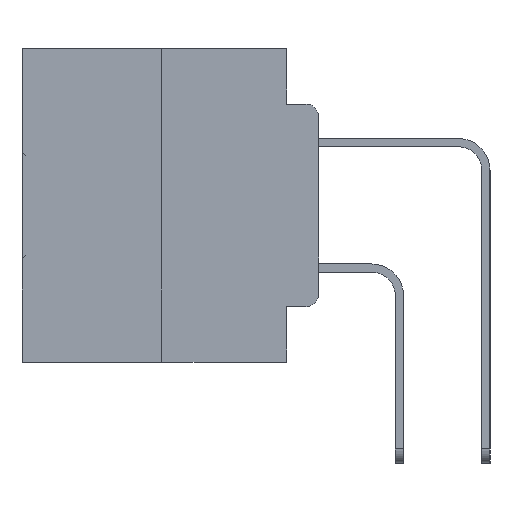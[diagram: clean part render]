
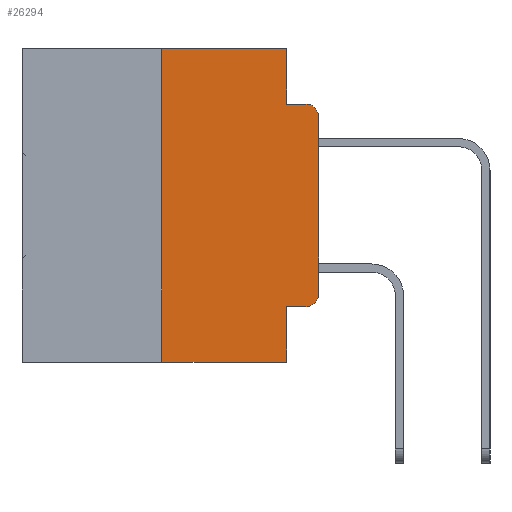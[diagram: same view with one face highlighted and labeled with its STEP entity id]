
A CAD part, left-side view. The second image highlights one B-rep face of the part: STEP entity #26294.
In plain terms, the highlighted planar face has unit normal (-1, 0, 0).
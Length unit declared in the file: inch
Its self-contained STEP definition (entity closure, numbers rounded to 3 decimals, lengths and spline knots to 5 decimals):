
#323 = CARTESIAN_POINT ( 'NONE',  ( 0., 0.02, -0.4115 ) ) ;
#711 = DIRECTION ( 'NONE',  ( 0., 0., -1. ) ) ;
#978 = VERTEX_POINT ( 'NONE', #22649 ) ;
#1404 = EDGE_CURVE ( 'NONE', #21995, #10503, #4610, .T. ) ;
#1432 = EDGE_CURVE ( 'NONE', #27067, #14574, #30393, .T. ) ;
#1796 = CARTESIAN_POINT ( 'NONE',  ( 0., 0.02, -0.3915 ) ) ;
#3207 = ORIENTED_EDGE ( 'NONE', *, *, #8226, .T. ) ;
#3226 = PLANE ( 'NONE',  #10144 ) ;
#4216 = DIRECTION ( 'NONE',  ( 0., -1., 0. ) ) ;
#4441 = DIRECTION ( 'NONE',  ( 0., 0., -1. ) ) ;
#4610 = LINE ( 'NONE', #26064, #17770 ) ;
#4712 = DIRECTION ( 'NONE',  ( 0., 0., -1. ) ) ;
#5640 = CARTESIAN_POINT ( 'NONE',  ( 0., 0., 0. ) ) ;
#6127 = ORIENTED_EDGE ( 'NONE', *, *, #20024, .F. ) ;
#6756 = CARTESIAN_POINT ( 'NONE',  ( 0., 0.473, 0. ) ) ;
#6758 = VECTOR ( 'NONE', #10884, 39.37008 ) ;
#6919 = VECTOR ( 'NONE', #30188, 39.37008 ) ;
#8086 = CARTESIAN_POINT ( 'NONE',  ( 0., 0.25, -0.5 ) ) ;
#8226 = EDGE_CURVE ( 'NONE', #978, #9316, #20683, .T. ) ;
#9015 = CARTESIAN_POINT ( 'NONE',  ( 0., 0.051, -0.4115 ) ) ;
#9114 = CIRCLE ( 'NONE', #15285, 0.02 ) ;
#9316 = VERTEX_POINT ( 'NONE', #19283 ) ;
#9957 = CARTESIAN_POINT ( 'NONE',  ( 0., 0.051, 0. ) ) ;
#10144 = AXIS2_PLACEMENT_3D ( 'NONE', #31971, #16475, #711 ) ;
#10295 = EDGE_CURVE ( 'NONE', #32346, #23845, #12346, .T. ) ;
#10503 = VERTEX_POINT ( 'NONE', #24082 ) ;
#10884 = DIRECTION ( 'NONE',  ( 0., 0., 1. ) ) ;
#10976 = EDGE_CURVE ( 'NONE', #27067, #10503, #20501, .T. ) ;
#11016 = CIRCLE ( 'NONE', #32434, 0.02 ) ;
#11503 = EDGE_CURVE ( 'NONE', #14574, #978, #11016, .T. ) ;
#11530 = VECTOR ( 'NONE', #15463, 39.37008 ) ;
#12202 = DIRECTION ( 'NONE',  ( 0., -1., 0. ) ) ;
#12247 = CARTESIAN_POINT ( 'NONE',  ( 0., 0.051, -0.4115 ) ) ;
#12346 = LINE ( 'NONE', #12783, #11530 ) ;
#12783 = CARTESIAN_POINT ( 'NONE',  ( 0., 0.051, -0.0885 ) ) ;
#13307 = CARTESIAN_POINT ( 'NONE',  ( 0., 0.051, -0.0885 ) ) ;
#13418 = DIRECTION ( 'NONE',  ( 0., -1., 0. ) ) ;
#13510 = VECTOR ( 'NONE', #33068, 39.37008 ) ;
#14574 = VERTEX_POINT ( 'NONE', #323 ) ;
#15016 = CARTESIAN_POINT ( 'NONE',  ( 0., 0.02, -0.1085 ) ) ;
#15285 = AXIS2_PLACEMENT_3D ( 'NONE', #15016, #33126, #17650 ) ;
#15463 = DIRECTION ( 'NONE',  ( 0., -1., 0. ) ) ;
#16025 = LINE ( 'NONE', #30500, #13510 ) ;
#16475 = DIRECTION ( 'NONE',  ( 1., 0., 0. ) ) ;
#17600 = EDGE_CURVE ( 'NONE', #19853, #32346, #16025, .T. ) ;
#17650 = DIRECTION ( 'NONE',  ( 0., 0., -1. ) ) ;
#17770 = VECTOR ( 'NONE', #13418, 39.37008 ) ;
#17836 = EDGE_LOOP ( 'NONE', ( #3207, #32586, #27341, #31395, #6127, #18043, #33420, #24558, #33019, #31031 ) ) ;
#18043 = ORIENTED_EDGE ( 'NONE', *, *, #20484, .F. ) ;
#19283 = CARTESIAN_POINT ( 'NONE',  ( 0., 0., -0.1085 ) ) ;
#19693 = VECTOR ( 'NONE', #4712, 39.37008 ) ;
#19853 = VERTEX_POINT ( 'NONE', #26862 ) ;
#20024 = EDGE_CURVE ( 'NONE', #28756, #19853, #22501, .T. ) ;
#20165 = DIRECTION ( 'NONE',  ( -1., 0., 0. ) ) ;
#20484 = EDGE_CURVE ( 'NONE', #21995, #28756, #20832, .T. ) ;
#20501 = LINE ( 'NONE', #9957, #19693 ) ;
#20683 = LINE ( 'NONE', #5640, #6758 ) ;
#20832 = LINE ( 'NONE', #27577, #6919 ) ;
#20863 = VECTOR ( 'NONE', #4216, 39.37008 ) ;
#21995 = VERTEX_POINT ( 'NONE', #8086 ) ;
#22501 = LINE ( 'NONE', #6756, #20863 ) ;
#22649 = CARTESIAN_POINT ( 'NONE',  ( 0., 0., -0.3915 ) ) ;
#23845 = VERTEX_POINT ( 'NONE', #33344 ) ;
#23906 = FACE_OUTER_BOUND ( 'NONE', #17836, .T. ) ;
#24082 = CARTESIAN_POINT ( 'NONE',  ( 0., 0.051, -0.5 ) ) ;
#24326 = VECTOR ( 'NONE', #12202, 39.37008 ) ;
#24558 = ORIENTED_EDGE ( 'NONE', *, *, #10976, .F. ) ;
#26064 = CARTESIAN_POINT ( 'NONE',  ( 0., 0.473, -0.5 ) ) ;
#26294 = ADVANCED_FACE ( 'NONE', ( #23906 ), #3226, .F. ) ;
#26862 = CARTESIAN_POINT ( 'NONE',  ( 0., 0.051, 0. ) ) ;
#27067 = VERTEX_POINT ( 'NONE', #9015 ) ;
#27240 = EDGE_CURVE ( 'NONE', #9316, #23845, #9114, .T. ) ;
#27341 = ORIENTED_EDGE ( 'NONE', *, *, #10295, .F. ) ;
#27577 = CARTESIAN_POINT ( 'NONE',  ( 0., 0.25, 0. ) ) ;
#28756 = VERTEX_POINT ( 'NONE', #31824 ) ;
#30188 = DIRECTION ( 'NONE',  ( 0., 0., 1. ) ) ;
#30393 = LINE ( 'NONE', #12247, #24326 ) ;
#30500 = CARTESIAN_POINT ( 'NONE',  ( 0., 0.051, 0. ) ) ;
#31031 = ORIENTED_EDGE ( 'NONE', *, *, #11503, .T. ) ;
#31395 = ORIENTED_EDGE ( 'NONE', *, *, #17600, .F. ) ;
#31824 = CARTESIAN_POINT ( 'NONE',  ( 0., 0.25, 0. ) ) ;
#31971 = CARTESIAN_POINT ( 'NONE',  ( 0., 0.473, 0. ) ) ;
#32346 = VERTEX_POINT ( 'NONE', #13307 ) ;
#32434 = AXIS2_PLACEMENT_3D ( 'NONE', #1796, #20165, #4441 ) ;
#32586 = ORIENTED_EDGE ( 'NONE', *, *, #27240, .T. ) ;
#33019 = ORIENTED_EDGE ( 'NONE', *, *, #1432, .T. ) ;
#33068 = DIRECTION ( 'NONE',  ( 0., 0., -1. ) ) ;
#33126 = DIRECTION ( 'NONE',  ( -1., 0., 0. ) ) ;
#33344 = CARTESIAN_POINT ( 'NONE',  ( 0., 0.02, -0.0885 ) ) ;
#33420 = ORIENTED_EDGE ( 'NONE', *, *, #1404, .T. ) ;
